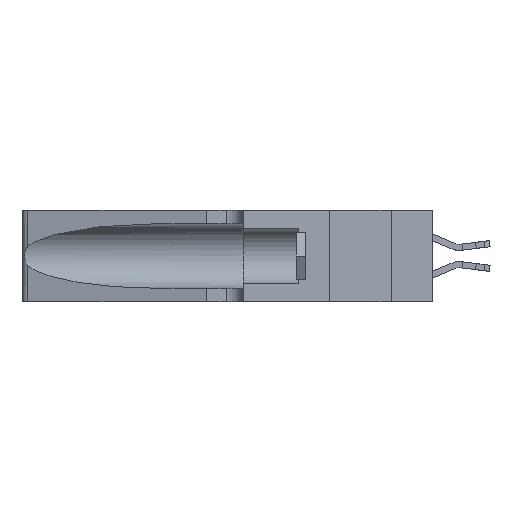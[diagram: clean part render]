
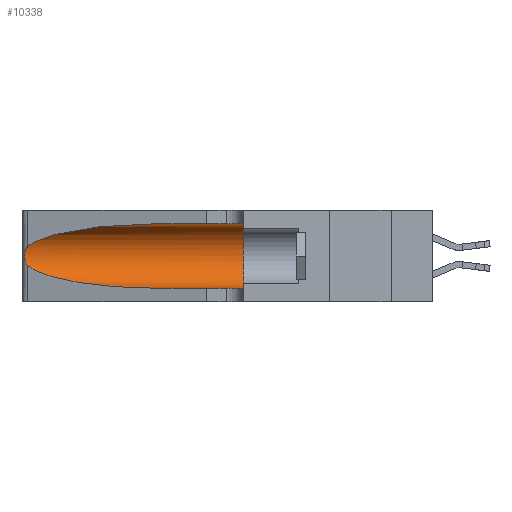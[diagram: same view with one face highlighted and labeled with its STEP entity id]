
A CAD part, left-side view. The second image highlights one B-rep face of the part: STEP entity #10338.
In plain terms, the highlighted cylindrical face has radius 3.308 mm (diameter 6.617 mm), a partial arc.
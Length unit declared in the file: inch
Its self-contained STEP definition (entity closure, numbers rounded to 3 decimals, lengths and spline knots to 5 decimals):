
#362 = VECTOR ( 'NONE', #510, 39.37008 ) ;
#510 = DIRECTION ( 'NONE',  ( 0., -1., 0. ) ) ;
#1870 = CARTESIAN_POINT ( 'NONE',  ( 0.1305, 0.72297, 0.31525 ) ) ;
#2568 = CARTESIAN_POINT ( 'NONE',  ( 0.26075, 1.23896, 0.178 ) ) ;
#2732 = CARTESIAN_POINT ( 'NONE',  ( 0.25487, 1.22718, 0.22369 ) ) ;
#3131 = EDGE_CURVE ( 'NONE', #14284, #22467, #15739, .T. ) ;
#3248 = EDGE_LOOP ( 'NONE', ( #6910, #10760, #10956, #6241, #20004, #12711 ) ) ;
#3311 = CARTESIAN_POINT ( 'NONE',  ( 0.18966, 0.96281, 0.31525 ) ) ;
#3723 = CARTESIAN_POINT ( 'NONE',  ( 0.1305, 1.61858, 0.05475 ) ) ;
#4024 = DIRECTION ( 'NONE',  ( 0., -1., 0. ) ) ;
#4443 = CARTESIAN_POINT ( 'NONE',  ( 0.25789, 1.23486, 0.15765 ) ) ;
#4608 = CARTESIAN_POINT ( 'NONE',  ( 0.25787, 1.23484, 0.2124 ) ) ;
#4652 = CARTESIAN_POINT ( 'NONE',  ( 0.1305, 0.35, 0.31525 ) ) ;
#4774 = LINE ( 'NONE', #9963, #362 ) ;
#5003 = VECTOR ( 'NONE', #4024, 39.37008 ) ;
#5687 = DIRECTION ( 'NONE',  ( 0., 0., 1. ) ) ;
#6225 = CARTESIAN_POINT ( 'NONE',  ( 0.25555, 1.22994, 0.2215 ) ) ;
#6241 = ORIENTED_EDGE ( 'NONE', *, *, #20092, .T. ) ;
#6311 = CARTESIAN_POINT ( 'NONE',  ( 0.26018, 1.23835, 0.19895 ) ) ;
#6472 =( BOUNDED_CURVE ( )  B_SPLINE_CURVE ( 3, ( #17753, #21760, #16210, #15971 ),
 .UNSPECIFIED., .F., .F. ) 
 B_SPLINE_CURVE_WITH_KNOTS ( ( 4, 4 ),
 ( 3.44316, 4.71239 ),
 .UNSPECIFIED. ) 
 CURVE ( )  GEOMETRIC_REPRESENTATION_ITEM ( )  RATIONAL_B_SPLINE_CURVE ( ( 1., 0.87, 0.87, 1. ) ) 
 REPRESENTATION_ITEM ( '' )  );
#6551 = CARTESIAN_POINT ( 'NONE',  ( 0.26075, 1.23896, 0.19203 ) ) ;
#6910 = ORIENTED_EDGE ( 'NONE', *, *, #16603, .T. ) ;
#6952 = DIRECTION ( 'NONE',  ( 0., -1., 0. ) ) ;
#7836 = CARTESIAN_POINT ( 'NONE',  ( 0.1305, 0.72297, 0.05475 ) ) ;
#8139 = CARTESIAN_POINT ( 'NONE',  ( 0.25555, 1.22993, 0.14849 ) ) ;
#8147 = FACE_OUTER_BOUND ( 'NONE', #3248, .T. ) ;
#8358 = CARTESIAN_POINT ( 'NONE',  ( 0.26017, 1.23833, 0.17102 ) ) ;
#8705 = VERTEX_POINT ( 'NONE', #7836 ) ;
#9084 = EDGE_CURVE ( 'NONE', #12259, #10650, #10195, .T. ) ;
#9340 = DIRECTION ( 'NONE',  ( 0., 1., 0. ) ) ;
#9514 = CARTESIAN_POINT ( 'NONE',  ( 0.1305, 0.35, 0.185 ) ) ;
#9946 = CARTESIAN_POINT ( 'NONE',  ( 0.25487, 1.22718, 0.22369 ) ) ;
#9963 = CARTESIAN_POINT ( 'NONE',  ( 0.1305, 1.61858, 0.31525 ) ) ;
#10195 = CIRCLE ( 'NONE', #23714, 0.13025 ) ;
#10338 = ADVANCED_FACE ( 'NONE', ( #8147 ), #22253, .F. ) ;
#10373 = CARTESIAN_POINT ( 'NONE',  ( 0.25487, 1.22718, 0.14631 ) ) ;
#10522 = CARTESIAN_POINT ( 'NONE',  ( 0.1305, 1.61858, 0.185 ) ) ;
#10650 = VERTEX_POINT ( 'NONE', #13907 ) ;
#10760 = ORIENTED_EDGE ( 'NONE', *, *, #3131, .T. ) ;
#10956 = ORIENTED_EDGE ( 'NONE', *, *, #12918, .T. ) ;
#11953 = AXIS2_PLACEMENT_3D ( 'NONE', #10522, #6952, #19838 ) ;
#12179 = CARTESIAN_POINT ( 'NONE',  ( 0.2373, 1.15595, 0.28018 ) ) ;
#12259 = VERTEX_POINT ( 'NONE', #4652 ) ;
#12711 = ORIENTED_EDGE ( 'NONE', *, *, #19211, .F. ) ;
#12918 = EDGE_CURVE ( 'NONE', #22467, #8705, #6472, .T. ) ;
#13907 = CARTESIAN_POINT ( 'NONE',  ( 0.1305, 0.35, 0.05475 ) ) ;
#14284 = VERTEX_POINT ( 'NONE', #9946 ) ;
#15444 = CARTESIAN_POINT ( 'NONE',  ( 0.25856, 1.23593, 0.16098 ) ) ;
#15620 = CARTESIAN_POINT ( 'NONE',  ( 0.25639, 1.23184, 0.21858 ) ) ;
#15739 = B_SPLINE_CURVE_WITH_KNOTS ( 'NONE', 3,
 ( #2732, #6225, #15620, #4608, #19118, #6311, #6551, #2568, #8358, #15444, #4443, #17320, #8139, #17405 ),
 .UNSPECIFIED., .F., .F.,
 ( 4, 2, 2, 2, 2, 2, 4 ),
 ( 0., 0.00027, 0.00053, 0.00107, 0.0016, 0.00187, 0.00214 ),
 .UNSPECIFIED. ) ;
#15971 = CARTESIAN_POINT ( 'NONE',  ( 0.1305, 0.72297, 0.05475 ) ) ;
#16210 = CARTESIAN_POINT ( 'NONE',  ( 0.18966, 0.96281, 0.05475 ) ) ;
#16603 = EDGE_CURVE ( 'NONE', #18948, #14284, #21792, .T. ) ;
#17320 = CARTESIAN_POINT ( 'NONE',  ( 0.25639, 1.23186, 0.15144 ) ) ;
#17405 = CARTESIAN_POINT ( 'NONE',  ( 0.25487, 1.22718, 0.14631 ) ) ;
#17753 = CARTESIAN_POINT ( 'NONE',  ( 0.25487, 1.22718, 0.14631 ) ) ;
#18948 = VERTEX_POINT ( 'NONE', #1870 ) ;
#19118 = CARTESIAN_POINT ( 'NONE',  ( 0.25854, 1.2359, 0.20912 ) ) ;
#19211 = EDGE_CURVE ( 'NONE', #18948, #12259, #4774, .T. ) ;
#19838 = DIRECTION ( 'NONE',  ( 0., 0., -1. ) ) ;
#20004 = ORIENTED_EDGE ( 'NONE', *, *, #9084, .F. ) ;
#20092 = EDGE_CURVE ( 'NONE', #8705, #10650, #21437, .T. ) ;
#21437 = LINE ( 'NONE', #3723, #5003 ) ;
#21760 = CARTESIAN_POINT ( 'NONE',  ( 0.2373, 1.15595, 0.08982 ) ) ;
#21792 =( BOUNDED_CURVE ( )  B_SPLINE_CURVE ( 3, ( #23547, #3311, #12179, #23408 ),
 .UNSPECIFIED., .F., .F. ) 
 B_SPLINE_CURVE_WITH_KNOTS ( ( 4, 4 ),
 ( 1.5708, 2.84003 ),
 .UNSPECIFIED. ) 
 CURVE ( )  GEOMETRIC_REPRESENTATION_ITEM ( )  RATIONAL_B_SPLINE_CURVE ( ( 1., 0.87, 0.87, 1. ) ) 
 REPRESENTATION_ITEM ( '' )  );
#22253 = CYLINDRICAL_SURFACE ( 'NONE', #11953, 0.13025 ) ;
#22467 = VERTEX_POINT ( 'NONE', #10373 ) ;
#23408 = CARTESIAN_POINT ( 'NONE',  ( 0.25487, 1.22718, 0.22369 ) ) ;
#23547 = CARTESIAN_POINT ( 'NONE',  ( 0.1305, 0.72297, 0.31525 ) ) ;
#23714 = AXIS2_PLACEMENT_3D ( 'NONE', #9514, #9340, #5687 ) ;
